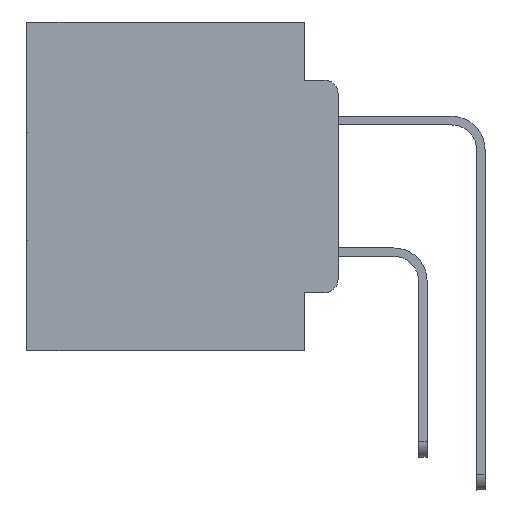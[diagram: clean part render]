
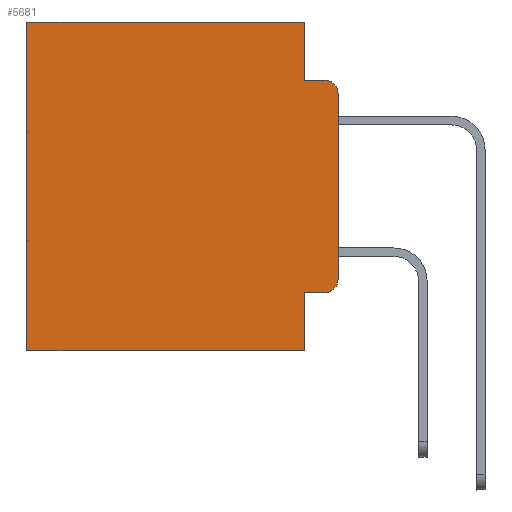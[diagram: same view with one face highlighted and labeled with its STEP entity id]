
A CAD part, left-side view. The second image highlights one B-rep face of the part: STEP entity #5681.
In plain terms, the highlighted planar face has unit normal (-1, 0, 0).
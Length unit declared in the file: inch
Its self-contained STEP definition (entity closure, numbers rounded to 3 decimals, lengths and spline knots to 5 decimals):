
#575 = CARTESIAN_POINT ( 'NONE',  ( 0.298, 0.051, 0. ) ) ;
#985 = AXIS2_PLACEMENT_3D ( 'NONE', #16007, #1290, #10603 ) ;
#1170 = PLANE ( 'NONE',  #16538 ) ;
#1290 = DIRECTION ( 'NONE',  ( -1., 0., 0. ) ) ;
#1325 = DIRECTION ( 'NONE',  ( 1., 0., 0. ) ) ;
#1556 = EDGE_CURVE ( 'NONE', #31020, #2630, #21968, .T. ) ;
#2349 = AXIS2_PLACEMENT_3D ( 'NONE', #21358, #14127, #31124 ) ;
#2396 = ORIENTED_EDGE ( 'NONE', *, *, #14873, .T. ) ;
#2630 = VERTEX_POINT ( 'NONE', #13628 ) ;
#2842 = EDGE_CURVE ( 'NONE', #19580, #29074, #10584, .T. ) ;
#4100 = CARTESIAN_POINT ( 'NONE',  ( 0.298, 0.051, 0. ) ) ;
#5017 = EDGE_CURVE ( 'NONE', #7678, #17796, #27792, .T. ) ;
#5410 = ORIENTED_EDGE ( 'NONE', *, *, #2842, .T. ) ;
#5429 = LINE ( 'NONE', #4100, #10943 ) ;
#5592 = CARTESIAN_POINT ( 'NONE',  ( 0.298, 0.473, 0. ) ) ;
#5681 = ADVANCED_FACE ( 'NONE', ( #8532 ), #1170, .F. ) ;
#7167 = CARTESIAN_POINT ( 'NONE',  ( 0.298, 0., -0.1085 ) ) ;
#7319 = LINE ( 'NONE', #24795, #12998 ) ;
#7450 = CARTESIAN_POINT ( 'NONE',  ( 0.298, 0., 0. ) ) ;
#7507 = CARTESIAN_POINT ( 'NONE',  ( 0.298, 0.051, -0.5 ) ) ;
#7678 = VERTEX_POINT ( 'NONE', #12867 ) ;
#7824 = DIRECTION ( 'NONE',  ( 0., -1., 0. ) ) ;
#8530 = CARTESIAN_POINT ( 'NONE',  ( 0.298, 0., -0.5 ) ) ;
#8532 = FACE_OUTER_BOUND ( 'NONE', #11620, .T. ) ;
#9649 = VERTEX_POINT ( 'NONE', #26433 ) ;
#10041 = LINE ( 'NONE', #7450, #27836 ) ;
#10551 = ORIENTED_EDGE ( 'NONE', *, *, #1556, .T. ) ;
#10584 = LINE ( 'NONE', #5592, #17294 ) ;
#10603 = DIRECTION ( 'NONE',  ( 0., 0., -1. ) ) ;
#10943 = VECTOR ( 'NONE', #18828, 39.37008 ) ;
#11457 = CARTESIAN_POINT ( 'NONE',  ( 0.298, 0.473, 0. ) ) ;
#11620 = EDGE_LOOP ( 'NONE', ( #16175, #10551, #28169, #19605, #2396, #5410, #15079, #25227, #26045, #30553 ) ) ;
#12867 = CARTESIAN_POINT ( 'NONE',  ( 0.298, 0.051, 0. ) ) ;
#12998 = VECTOR ( 'NONE', #19642, 39.37008 ) ;
#13322 = LINE ( 'NONE', #8530, #23611 ) ;
#13628 = CARTESIAN_POINT ( 'NONE',  ( 0.298, 0.02, -0.0885 ) ) ;
#14127 = DIRECTION ( 'NONE',  ( -1., 0., 0. ) ) ;
#14452 = VECTOR ( 'NONE', #7824, 39.37008 ) ;
#14873 = EDGE_CURVE ( 'NONE', #7678, #19580, #10041, .T. ) ;
#14909 = VECTOR ( 'NONE', #27827, 39.37008 ) ;
#15079 = ORIENTED_EDGE ( 'NONE', *, *, #16039, .F. ) ;
#15140 = DIRECTION ( 'NONE',  ( 0., 1., 0. ) ) ;
#15632 = CIRCLE ( 'NONE', #2349, 0.02 ) ;
#16007 = CARTESIAN_POINT ( 'NONE',  ( 0.298, 0.02, -0.1085 ) ) ;
#16039 = EDGE_CURVE ( 'NONE', #26484, #29074, #13322, .T. ) ;
#16041 = DIRECTION ( 'NONE',  ( 0., 1., 0. ) ) ;
#16114 = LINE ( 'NONE', #18049, #14909 ) ;
#16175 = ORIENTED_EDGE ( 'NONE', *, *, #20640, .F. ) ;
#16538 = AXIS2_PLACEMENT_3D ( 'NONE', #20706, #1325, #30491 ) ;
#16795 = EDGE_CURVE ( 'NONE', #17796, #2630, #17755, .T. ) ;
#17038 = VERTEX_POINT ( 'NONE', #30238 ) ;
#17294 = VECTOR ( 'NONE', #17631, 39.37008 ) ;
#17631 = DIRECTION ( 'NONE',  ( 0., 0., -1. ) ) ;
#17713 = VERTEX_POINT ( 'NONE', #27294 ) ;
#17755 = LINE ( 'NONE', #19976, #14452 ) ;
#17796 = VERTEX_POINT ( 'NONE', #29388 ) ;
#18049 = CARTESIAN_POINT ( 'NONE',  ( 0.298, 0.051, -0.4115 ) ) ;
#18828 = DIRECTION ( 'NONE',  ( 0., 0., -1. ) ) ;
#19580 = VERTEX_POINT ( 'NONE', #11457 ) ;
#19605 = ORIENTED_EDGE ( 'NONE', *, *, #5017, .F. ) ;
#19642 = DIRECTION ( 'NONE',  ( 0., 0., -1. ) ) ;
#19976 = CARTESIAN_POINT ( 'NONE',  ( 0.298, 0.051, -0.0885 ) ) ;
#20385 = EDGE_CURVE ( 'NONE', #9649, #26484, #5429, .T. ) ;
#20640 = EDGE_CURVE ( 'NONE', #31020, #17713, #7319, .T. ) ;
#20706 = CARTESIAN_POINT ( 'NONE',  ( 0.298, 0., 0. ) ) ;
#21358 = CARTESIAN_POINT ( 'NONE',  ( 0.298, 0.02, -0.3915 ) ) ;
#21968 = CIRCLE ( 'NONE', #985, 0.02 ) ;
#22705 = EDGE_CURVE ( 'NONE', #17038, #17713, #15632, .T. ) ;
#23145 = VECTOR ( 'NONE', #25236, 39.37008 ) ;
#23611 = VECTOR ( 'NONE', #16041, 39.37008 ) ;
#24795 = CARTESIAN_POINT ( 'NONE',  ( 0.298, 0., 0. ) ) ;
#25227 = ORIENTED_EDGE ( 'NONE', *, *, #20385, .F. ) ;
#25236 = DIRECTION ( 'NONE',  ( 0., 0., -1. ) ) ;
#25824 = CARTESIAN_POINT ( 'NONE',  ( 0.298, 0.473, -0.5 ) ) ;
#26045 = ORIENTED_EDGE ( 'NONE', *, *, #29967, .T. ) ;
#26433 = CARTESIAN_POINT ( 'NONE',  ( 0.298, 0.051, -0.4115 ) ) ;
#26484 = VERTEX_POINT ( 'NONE', #7507 ) ;
#27294 = CARTESIAN_POINT ( 'NONE',  ( 0.298, 0., -0.3915 ) ) ;
#27792 = LINE ( 'NONE', #575, #23145 ) ;
#27827 = DIRECTION ( 'NONE',  ( 0., -1., 0. ) ) ;
#27836 = VECTOR ( 'NONE', #15140, 39.37008 ) ;
#28169 = ORIENTED_EDGE ( 'NONE', *, *, #16795, .F. ) ;
#29074 = VERTEX_POINT ( 'NONE', #25824 ) ;
#29388 = CARTESIAN_POINT ( 'NONE',  ( 0.298, 0.051, -0.0885 ) ) ;
#29967 = EDGE_CURVE ( 'NONE', #9649, #17038, #16114, .T. ) ;
#30238 = CARTESIAN_POINT ( 'NONE',  ( 0.298, 0.02, -0.4115 ) ) ;
#30491 = DIRECTION ( 'NONE',  ( 0., 0., -1. ) ) ;
#30553 = ORIENTED_EDGE ( 'NONE', *, *, #22705, .T. ) ;
#31020 = VERTEX_POINT ( 'NONE', #7167 ) ;
#31124 = DIRECTION ( 'NONE',  ( 0., 0., -1. ) ) ;
